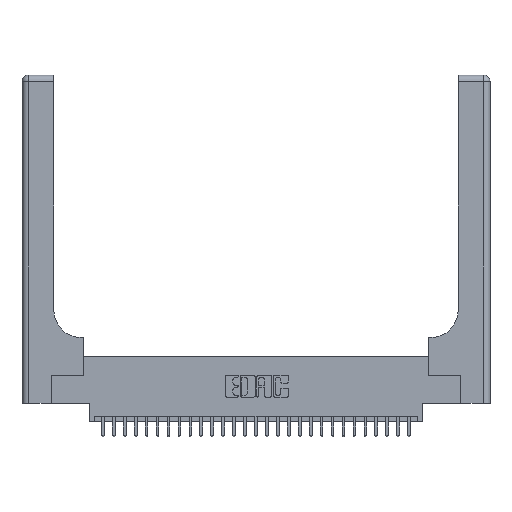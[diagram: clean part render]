
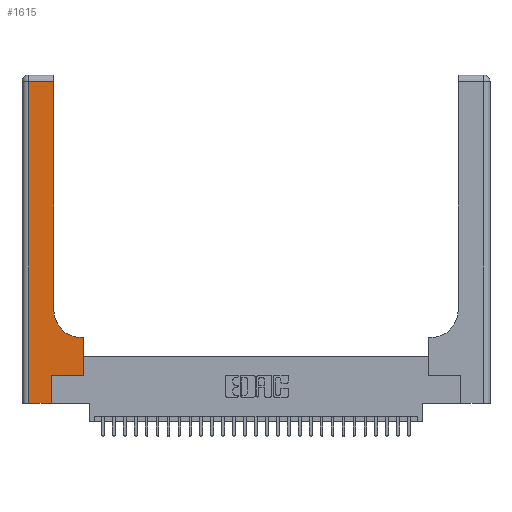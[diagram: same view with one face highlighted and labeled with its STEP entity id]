
A CAD part, top view. The second image highlights one B-rep face of the part: STEP entity #1615.
In plain terms, the highlighted planar face has unit normal (0, 0, 1).
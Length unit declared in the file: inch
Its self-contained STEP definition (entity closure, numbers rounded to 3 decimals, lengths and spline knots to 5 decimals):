
#191 = EDGE_CURVE ( 'NONE', #4193, #13328, #23938, .T. ) ;
#520 = VERTEX_POINT ( 'NONE', #5744 ) ;
#1423 = CIRCLE ( 'NONE', #7713, 0.25 ) ;
#1466 = FACE_OUTER_BOUND ( 'NONE', #1592, .T. ) ;
#1526 = CARTESIAN_POINT ( 'NONE',  ( 0.2915, 0.6, 0.37 ) ) ;
#1592 = EDGE_LOOP ( 'NONE', ( #6573, #2649, #22589, #2768, #4572, #29534, #3297, #14882, #24755 ) ) ;
#1615 = ADVANCED_FACE ( 'NONE', ( #1466 ), #18940, .F. ) ;
#2649 = ORIENTED_EDGE ( 'NONE', *, *, #25132, .T. ) ;
#2768 = ORIENTED_EDGE ( 'NONE', *, *, #11325, .T. ) ;
#3174 = EDGE_CURVE ( 'NONE', #22893, #19616, #10008, .T. ) ;
#3283 = VERTEX_POINT ( 'NONE', #26517 ) ;
#3292 = CARTESIAN_POINT ( 'NONE',  ( 0.269, 0., 0.37 ) ) ;
#3297 = ORIENTED_EDGE ( 'NONE', *, *, #191, .T. ) ;
#3651 = LINE ( 'NONE', #1526, #21393 ) ;
#4193 = VERTEX_POINT ( 'NONE', #13792 ) ;
#4572 = ORIENTED_EDGE ( 'NONE', *, *, #3174, .T. ) ;
#4704 = LINE ( 'NONE', #6311, #17024 ) ;
#4841 = CARTESIAN_POINT ( 'NONE',  ( 0.06, 3., 0.37 ) ) ;
#5236 = CARTESIAN_POINT ( 'NONE',  ( 0.2915, 3., 0.37 ) ) ;
#5264 = DIRECTION ( 'NONE',  ( -1., 0., 0. ) ) ;
#5744 = CARTESIAN_POINT ( 'NONE',  ( 0.06, 2.94, 0.37 ) ) ;
#6311 = CARTESIAN_POINT ( 'NONE',  ( 0.269, 0.25, 0.37 ) ) ;
#6322 = VERTEX_POINT ( 'NONE', #11328 ) ;
#6573 = ORIENTED_EDGE ( 'NONE', *, *, #19904, .T. ) ;
#6882 = DIRECTION ( 'NONE',  ( 0., 1., 0. ) ) ;
#7168 = EDGE_CURVE ( 'NONE', #520, #6322, #24823, .T. ) ;
#7266 = DIRECTION ( 'NONE',  ( 0., 0., -1. ) ) ;
#7565 = DIRECTION ( 'NONE',  ( 0., 1., 0. ) ) ;
#7713 = AXIS2_PLACEMENT_3D ( 'NONE', #21137, #7266, #23460 ) ;
#9035 = LINE ( 'NONE', #21902, #14471 ) ;
#10008 = LINE ( 'NONE', #21654, #26960 ) ;
#10605 = CARTESIAN_POINT ( 'NONE',  ( 0.269, 0.25, 0.37 ) ) ;
#10797 = EDGE_CURVE ( 'NONE', #13328, #3283, #3651, .T. ) ;
#11325 = EDGE_CURVE ( 'NONE', #6322, #22893, #9035, .T. ) ;
#11328 = CARTESIAN_POINT ( 'NONE',  ( 0.06, 0., 0.37 ) ) ;
#11522 = EDGE_CURVE ( 'NONE', #19616, #4193, #4704, .T. ) ;
#12052 = DIRECTION ( 'NONE',  ( 0., 0., -1. ) ) ;
#13001 = DIRECTION ( 'NONE',  ( -1., 0., 0. ) ) ;
#13328 = VERTEX_POINT ( 'NONE', #15584 ) ;
#13792 = CARTESIAN_POINT ( 'NONE',  ( 0.5585, 0.25, 0.37 ) ) ;
#14471 = VECTOR ( 'NONE', #28701, 39.37008 ) ;
#14512 = VECTOR ( 'NONE', #7565, 39.37008 ) ;
#14668 = DIRECTION ( 'NONE',  ( 0., 1., 0. ) ) ;
#14882 = ORIENTED_EDGE ( 'NONE', *, *, #10797, .T. ) ;
#15239 = LINE ( 'NONE', #5236, #14512 ) ;
#15584 = CARTESIAN_POINT ( 'NONE',  ( 0.5585, 0.6, 0.37 ) ) ;
#17024 = VECTOR ( 'NONE', #29391, 39.37008 ) ;
#18708 = VECTOR ( 'NONE', #18790, 39.37008 ) ;
#18790 = DIRECTION ( 'NONE',  ( 0., -1., 0. ) ) ;
#18940 = PLANE ( 'NONE',  #22245 ) ;
#18973 = VERTEX_POINT ( 'NONE', #24580 ) ;
#19616 = VERTEX_POINT ( 'NONE', #10605 ) ;
#19904 = EDGE_CURVE ( 'NONE', #18973, #26811, #15239, .T. ) ;
#20745 = CARTESIAN_POINT ( 'NONE',  ( 0.5585, 0.25, 0.37 ) ) ;
#21137 = CARTESIAN_POINT ( 'NONE',  ( 0.5415, 0.85, 0.37 ) ) ;
#21280 = CARTESIAN_POINT ( 'NONE',  ( 0., 3., 0.37 ) ) ;
#21370 = CARTESIAN_POINT ( 'NONE',  ( 0.2915, 2.94, 0.37 ) ) ;
#21393 = VECTOR ( 'NONE', #13001, 39.37008 ) ;
#21455 = CARTESIAN_POINT ( 'NONE',  ( 0., 2.94, 0.37 ) ) ;
#21654 = CARTESIAN_POINT ( 'NONE',  ( 0.269, 0., 0.37 ) ) ;
#21902 = CARTESIAN_POINT ( 'NONE',  ( 0., 0., 0.37 ) ) ;
#22121 = EDGE_CURVE ( 'NONE', #3283, #18973, #1423, .T. ) ;
#22245 = AXIS2_PLACEMENT_3D ( 'NONE', #21280, #12052, #28188 ) ;
#22589 = ORIENTED_EDGE ( 'NONE', *, *, #7168, .T. ) ;
#22893 = VERTEX_POINT ( 'NONE', #3292 ) ;
#23460 = DIRECTION ( 'NONE',  ( 1., 0., 0. ) ) ;
#23938 = LINE ( 'NONE', #20745, #25373 ) ;
#24580 = CARTESIAN_POINT ( 'NONE',  ( 0.2915, 0.85, 0.37 ) ) ;
#24755 = ORIENTED_EDGE ( 'NONE', *, *, #22121, .T. ) ;
#24823 = LINE ( 'NONE', #4841, #18708 ) ;
#25132 = EDGE_CURVE ( 'NONE', #26811, #520, #27178, .T. ) ;
#25373 = VECTOR ( 'NONE', #6882, 39.37008 ) ;
#26454 = VECTOR ( 'NONE', #5264, 39.37008 ) ;
#26517 = CARTESIAN_POINT ( 'NONE',  ( 0.5415, 0.6, 0.37 ) ) ;
#26811 = VERTEX_POINT ( 'NONE', #21370 ) ;
#26960 = VECTOR ( 'NONE', #14668, 39.37008 ) ;
#27178 = LINE ( 'NONE', #21455, #26454 ) ;
#28188 = DIRECTION ( 'NONE',  ( -1., 0., 0. ) ) ;
#28701 = DIRECTION ( 'NONE',  ( 1., 0., 0. ) ) ;
#29391 = DIRECTION ( 'NONE',  ( 1., 0., 0. ) ) ;
#29534 = ORIENTED_EDGE ( 'NONE', *, *, #11522, .T. ) ;
